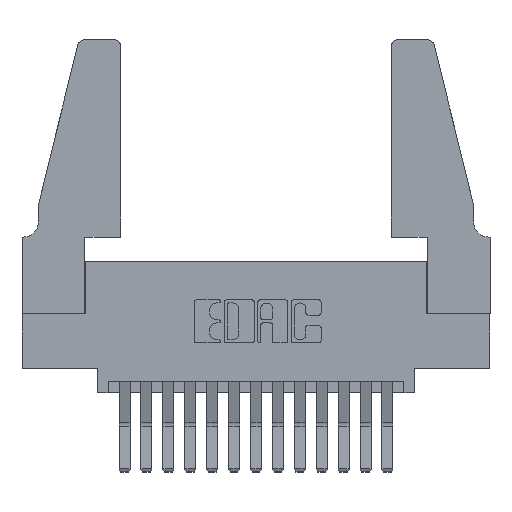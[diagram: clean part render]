
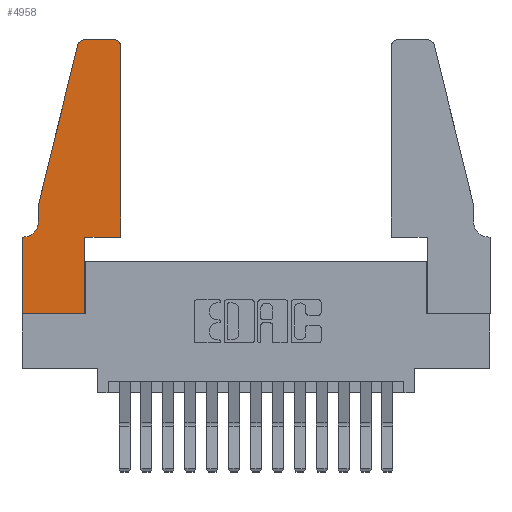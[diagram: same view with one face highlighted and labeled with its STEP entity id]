
A CAD part, top view. The second image highlights one B-rep face of the part: STEP entity #4958.
In plain terms, the highlighted planar face has unit normal (0, 0, 1).
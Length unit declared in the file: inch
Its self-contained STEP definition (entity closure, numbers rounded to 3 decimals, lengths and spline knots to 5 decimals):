
#53 = EDGE_CURVE ( 'NONE', #6540, #15874, #15536, .T. ) ;
#96 = ORIENTED_EDGE ( 'NONE', *, *, #15811, .T. ) ;
#181 = VERTEX_POINT ( 'NONE', #14047 ) ;
#264 = ORIENTED_EDGE ( 'NONE', *, *, #6416, .T. ) ;
#386 = DIRECTION ( 'NONE',  ( 0., -1., 0. ) ) ;
#433 = CARTESIAN_POINT ( 'NONE',  ( 0.0755, 0.5, 0.37 ) ) ;
#467 = CARTESIAN_POINT ( 'NONE',  ( 0., 0.35, 0.37 ) ) ;
#546 = CARTESIAN_POINT ( 'NONE',  ( 0.25487, 1.22718, 0.37 ) ) ;
#687 = VERTEX_POINT ( 'NONE', #546 ) ;
#732 = ORIENTED_EDGE ( 'NONE', *, *, #11796, .T. ) ;
#970 = CIRCLE ( 'NONE', #6660, 0.07 ) ;
#1487 = VERTEX_POINT ( 'NONE', #6211 ) ;
#1512 = DIRECTION ( 'NONE',  ( 1., 0., 0. ) ) ;
#1623 = CARTESIAN_POINT ( 'NONE',  ( 0.0755, 0.5, 0.37 ) ) ;
#1788 = VECTOR ( 'NONE', #386, 39.37008 ) ;
#2057 = DIRECTION ( 'NONE',  ( 1., 0., 0. ) ) ;
#2144 = CARTESIAN_POINT ( 'NONE',  ( 0., 0.35, 0.37 ) ) ;
#2255 = AXIS2_PLACEMENT_3D ( 'NONE', #6508, #2695, #1512 ) ;
#2298 = CIRCLE ( 'NONE', #5539, 0.03 ) ;
#2503 = VECTOR ( 'NONE', #10523, 39.37008 ) ;
#2615 = VERTEX_POINT ( 'NONE', #8103 ) ;
#2695 = DIRECTION ( 'NONE',  ( 0., 0., 1. ) ) ;
#2768 = VERTEX_POINT ( 'NONE', #8119 ) ;
#2971 = ORIENTED_EDGE ( 'NONE', *, *, #14341, .T. ) ;
#3088 = DIRECTION ( 'NONE',  ( 0., 1., 0. ) ) ;
#3248 = DIRECTION ( 'NONE',  ( 1., 0., 0. ) ) ;
#3391 = VECTOR ( 'NONE', #14932, 39.37008 ) ;
#3416 = VERTEX_POINT ( 'NONE', #7413 ) ;
#3731 = VECTOR ( 'NONE', #3248, 39.37008 ) ;
#3923 = ORIENTED_EDGE ( 'NONE', *, *, #4066, .T. ) ;
#4000 = ORIENTED_EDGE ( 'NONE', *, *, #5450, .T. ) ;
#4066 = EDGE_CURVE ( 'NONE', #1487, #6493, #6014, .T. ) ;
#4471 = VERTEX_POINT ( 'NONE', #10696 ) ;
#4958 = ADVANCED_FACE ( 'NONE', ( #15923 ), #5334, .T. ) ;
#5140 = DIRECTION ( 'NONE',  ( 1., 0., 0. ) ) ;
#5334 = PLANE ( 'NONE',  #13686 ) ;
#5450 = EDGE_CURVE ( 'NONE', #2615, #687, #8172, .T. ) ;
#5539 = AXIS2_PLACEMENT_3D ( 'NONE', #7597, #12789, #5140 ) ;
#5748 = DIRECTION ( 'NONE',  ( 0., 0., 1. ) ) ;
#6014 = LINE ( 'NONE', #1623, #1788 ) ;
#6211 = CARTESIAN_POINT ( 'NONE',  ( 0.0755, 0.5, 0.37 ) ) ;
#6322 = LINE ( 'NONE', #10363, #2503 ) ;
#6416 = EDGE_CURVE ( 'NONE', #4471, #3416, #16251, .T. ) ;
#6493 = VERTEX_POINT ( 'NONE', #16273 ) ;
#6508 = CARTESIAN_POINT ( 'NONE',  ( 0.284, 1.22, 0.37 ) ) ;
#6540 = VERTEX_POINT ( 'NONE', #2144 ) ;
#6660 = AXIS2_PLACEMENT_3D ( 'NONE', #11932, #6732, #11812 ) ;
#6732 = DIRECTION ( 'NONE',  ( 0., 0., -1. ) ) ;
#6908 = CARTESIAN_POINT ( 'NONE',  ( 0.2865, 0.35, 0.37 ) ) ;
#7413 = CARTESIAN_POINT ( 'NONE',  ( 0.2865, 0.35, 0.37 ) ) ;
#7594 = VECTOR ( 'NONE', #16385, 39.37008 ) ;
#7597 = CARTESIAN_POINT ( 'NONE',  ( 0.4205, 1.22, 0.37 ) ) ;
#7997 = VECTOR ( 'NONE', #9408, 39.37008 ) ;
#8103 = CARTESIAN_POINT ( 'NONE',  ( 0.284, 1.25, 0.37 ) ) ;
#8119 = CARTESIAN_POINT ( 'NONE',  ( 0.4505, 0.35, 0.37 ) ) ;
#8172 = CIRCLE ( 'NONE', #2255, 0.03 ) ;
#8474 = CARTESIAN_POINT ( 'NONE',  ( 0., 0., 0.37 ) ) ;
#8737 = VECTOR ( 'NONE', #3088, 39.37008 ) ;
#9234 = EDGE_CURVE ( 'NONE', #13243, #11643, #2298, .T. ) ;
#9288 = CARTESIAN_POINT ( 'NONE',  ( 0.4205, 1.25, 0.37 ) ) ;
#9408 = DIRECTION ( 'NONE',  ( -0.239, -0.971, 0. ) ) ;
#9560 = VECTOR ( 'NONE', #15379, 39.37008 ) ;
#9618 = LINE ( 'NONE', #433, #7997 ) ;
#9644 = LINE ( 'NONE', #12943, #3391 ) ;
#10286 = ORIENTED_EDGE ( 'NONE', *, *, #9234, .T. ) ;
#10363 = CARTESIAN_POINT ( 'NONE',  ( 0.0755, 0.35, 0.37 ) ) ;
#10422 = ORIENTED_EDGE ( 'NONE', *, *, #12564, .T. ) ;
#10523 = DIRECTION ( 'NONE',  ( -1., 0., 0. ) ) ;
#10675 = DIRECTION ( 'NONE',  ( 1., 0., 0. ) ) ;
#10696 = CARTESIAN_POINT ( 'NONE',  ( 0.2865, 0., 0.37 ) ) ;
#11333 = CARTESIAN_POINT ( 'NONE',  ( 0., 0., 0.37 ) ) ;
#11643 = VERTEX_POINT ( 'NONE', #9288 ) ;
#11796 = EDGE_CURVE ( 'NONE', #2768, #13243, #9644, .T. ) ;
#11812 = DIRECTION ( 'NONE',  ( -1., 0., 0. ) ) ;
#11932 = CARTESIAN_POINT ( 'NONE',  ( 0.0055, 0.42, 0.37 ) ) ;
#12225 = CARTESIAN_POINT ( 'NONE',  ( 0.4505, 1.22, 0.37 ) ) ;
#12541 = LINE ( 'NONE', #15435, #9560 ) ;
#12564 = EDGE_CURVE ( 'NONE', #3416, #2768, #15710, .T. ) ;
#12789 = DIRECTION ( 'NONE',  ( 0., 0., 1. ) ) ;
#12851 = ORIENTED_EDGE ( 'NONE', *, *, #12897, .T. ) ;
#12897 = EDGE_CURVE ( 'NONE', #181, #6540, #6322, .T. ) ;
#12943 = CARTESIAN_POINT ( 'NONE',  ( 0.4505, 0.35, 0.37 ) ) ;
#13159 = VECTOR ( 'NONE', #2057, 39.37008 ) ;
#13243 = VERTEX_POINT ( 'NONE', #12225 ) ;
#13686 = AXIS2_PLACEMENT_3D ( 'NONE', #467, #5748, #10675 ) ;
#14047 = CARTESIAN_POINT ( 'NONE',  ( 0.0055, 0.35, 0.37 ) ) ;
#14341 = EDGE_CURVE ( 'NONE', #687, #1487, #9618, .T. ) ;
#14557 = ORIENTED_EDGE ( 'NONE', *, *, #14949, .T. ) ;
#14735 = CARTESIAN_POINT ( 'NONE',  ( 0., 0., 0.37 ) ) ;
#14810 = EDGE_LOOP ( 'NONE', ( #14880, #4000, #2971, #3923, #14557, #12851, #16125, #96, #264, #10422, #732, #10286 ) ) ;
#14880 = ORIENTED_EDGE ( 'NONE', *, *, #16103, .T. ) ;
#14932 = DIRECTION ( 'NONE',  ( 0., 1., 0. ) ) ;
#14949 = EDGE_CURVE ( 'NONE', #6493, #181, #970, .T. ) ;
#15379 = DIRECTION ( 'NONE',  ( -1., 0., 0. ) ) ;
#15435 = CARTESIAN_POINT ( 'NONE',  ( 0.2605, 1.25, 0.37 ) ) ;
#15536 = LINE ( 'NONE', #11333, #7594 ) ;
#15710 = LINE ( 'NONE', #16028, #13159 ) ;
#15811 = EDGE_CURVE ( 'NONE', #15874, #4471, #16473, .T. ) ;
#15874 = VERTEX_POINT ( 'NONE', #14735 ) ;
#15923 = FACE_OUTER_BOUND ( 'NONE', #14810, .T. ) ;
#16028 = CARTESIAN_POINT ( 'NONE',  ( 0.4505, 0.35, 0.37 ) ) ;
#16103 = EDGE_CURVE ( 'NONE', #11643, #2615, #12541, .T. ) ;
#16125 = ORIENTED_EDGE ( 'NONE', *, *, #53, .T. ) ;
#16251 = LINE ( 'NONE', #6908, #8737 ) ;
#16273 = CARTESIAN_POINT ( 'NONE',  ( 0.0755, 0.42, 0.37 ) ) ;
#16385 = DIRECTION ( 'NONE',  ( 0., -1., 0. ) ) ;
#16473 = LINE ( 'NONE', #8474, #3731 ) ;
